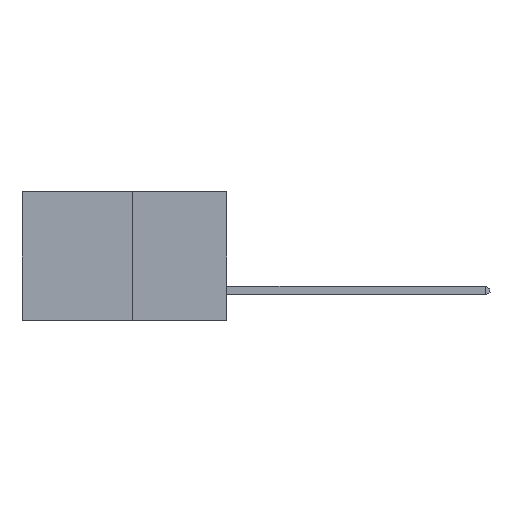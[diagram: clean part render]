
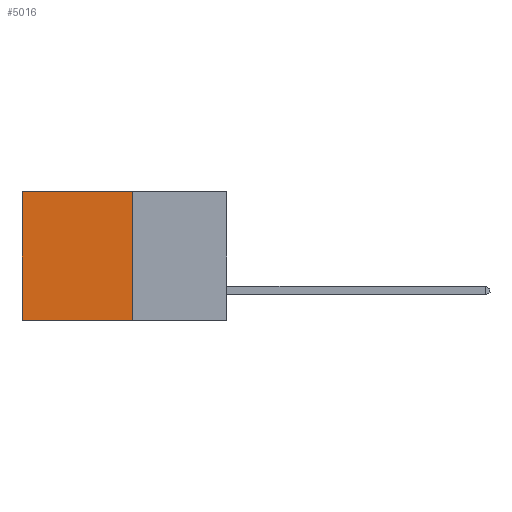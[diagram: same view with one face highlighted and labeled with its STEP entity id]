
A CAD part, left-side view. The second image highlights one B-rep face of the part: STEP entity #5016.
In plain terms, the highlighted planar face has unit normal (-1, 0, 0).
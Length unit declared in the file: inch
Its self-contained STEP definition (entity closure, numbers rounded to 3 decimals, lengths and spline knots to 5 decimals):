
#54 = EDGE_CURVE ( 'NONE', #3001, #9243, #2191, .T. ) ;
#179 = VECTOR ( 'NONE', #3843, 39.37008 ) ;
#382 = VECTOR ( 'NONE', #7962, 39.37008 ) ;
#489 = VECTOR ( 'NONE', #7489, 39.37008 ) ;
#1317 = CARTESIAN_POINT ( 'NONE',  ( 0.277, 0.27, 0. ) ) ;
#1649 = ORIENTED_EDGE ( 'NONE', *, *, #54, .T. ) ;
#2191 = LINE ( 'NONE', #7125, #179 ) ;
#2478 = LINE ( 'NONE', #5489, #489 ) ;
#2563 = EDGE_CURVE ( 'NONE', #9243, #8960, #8246, .T. ) ;
#3001 = VERTEX_POINT ( 'NONE', #1317 ) ;
#3198 = EDGE_CURVE ( 'NONE', #3001, #6483, #2478, .T. ) ;
#3371 = CARTESIAN_POINT ( 'NONE',  ( 0.277, 0.59, 0. ) ) ;
#3443 = DIRECTION ( 'NONE',  ( 0., 0., -1. ) ) ;
#3843 = DIRECTION ( 'NONE',  ( 0., 1., 0. ) ) ;
#3849 = VECTOR ( 'NONE', #6184, 39.37008 ) ;
#3881 = EDGE_CURVE ( 'NONE', #6483, #8960, #5794, .T. ) ;
#3888 = ORIENTED_EDGE ( 'NONE', *, *, #2563, .T. ) ;
#4455 = CARTESIAN_POINT ( 'NONE',  ( 0.277, 0.59, -0.37 ) ) ;
#4644 = DIRECTION ( 'NONE',  ( 1., 0., 0. ) ) ;
#4649 = CARTESIAN_POINT ( 'NONE',  ( 0.277, 0.27, -0.37 ) ) ;
#4656 = PLANE ( 'NONE',  #5344 ) ;
#4934 = EDGE_LOOP ( 'NONE', ( #3888, #6252, #6703, #1649 ) ) ;
#5016 = ADVANCED_FACE ( 'NONE', ( #9089 ), #4656, .F. ) ;
#5344 = AXIS2_PLACEMENT_3D ( 'NONE', #4649, #4644, #3443 ) ;
#5489 = CARTESIAN_POINT ( 'NONE',  ( 0.277, 0.27, -0.37 ) ) ;
#5738 = CARTESIAN_POINT ( 'NONE',  ( 0.277, 0.27, -0.37 ) ) ;
#5794 = LINE ( 'NONE', #5738, #3849 ) ;
#6184 = DIRECTION ( 'NONE',  ( 0., 1., 0. ) ) ;
#6252 = ORIENTED_EDGE ( 'NONE', *, *, #3881, .F. ) ;
#6483 = VERTEX_POINT ( 'NONE', #7617 ) ;
#6703 = ORIENTED_EDGE ( 'NONE', *, *, #3198, .F. ) ;
#7125 = CARTESIAN_POINT ( 'NONE',  ( 0.277, 0.27, 0. ) ) ;
#7307 = CARTESIAN_POINT ( 'NONE',  ( 0.277, 0.59, -0.37 ) ) ;
#7489 = DIRECTION ( 'NONE',  ( 0., 0., -1. ) ) ;
#7617 = CARTESIAN_POINT ( 'NONE',  ( 0.277, 0.27, -0.37 ) ) ;
#7962 = DIRECTION ( 'NONE',  ( 0., 0., -1. ) ) ;
#8246 = LINE ( 'NONE', #4455, #382 ) ;
#8960 = VERTEX_POINT ( 'NONE', #7307 ) ;
#9089 = FACE_OUTER_BOUND ( 'NONE', #4934, .T. ) ;
#9243 = VERTEX_POINT ( 'NONE', #3371 ) ;
